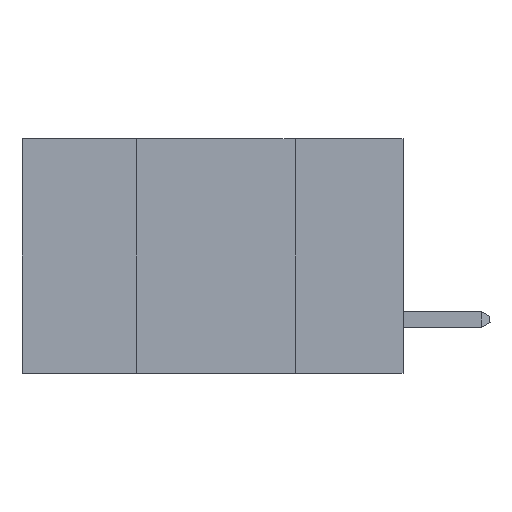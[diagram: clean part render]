
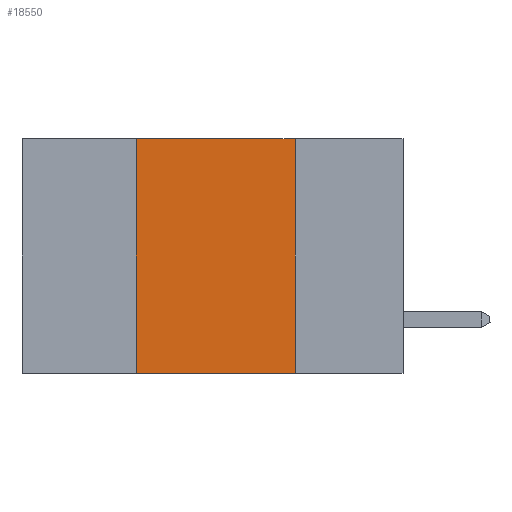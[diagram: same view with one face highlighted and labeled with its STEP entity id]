
A CAD part, left-side view. The second image highlights one B-rep face of the part: STEP entity #18550.
In plain terms, the highlighted planar face has unit normal (-1, 0, 0).
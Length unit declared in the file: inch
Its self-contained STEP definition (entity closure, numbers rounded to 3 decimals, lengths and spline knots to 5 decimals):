
#1432 = CARTESIAN_POINT ( 'NONE',  ( 0., 0.42, -0.37 ) ) ;
#1629 = LINE ( 'NONE', #10689, #16198 ) ;
#2350 = VECTOR ( 'NONE', #7795, 39.37008 ) ;
#4616 = FACE_OUTER_BOUND ( 'NONE', #24418, .T. ) ;
#4777 = DIRECTION ( 'NONE',  ( 0., -1., 0. ) ) ;
#5772 = CARTESIAN_POINT ( 'NONE',  ( 0., 0.17, 0. ) ) ;
#6080 = CARTESIAN_POINT ( 'NONE',  ( 0., 0.42, 0. ) ) ;
#7795 = DIRECTION ( 'NONE',  ( 0., 0., -1. ) ) ;
#7841 = VERTEX_POINT ( 'NONE', #17746 ) ;
#8073 = ORIENTED_EDGE ( 'NONE', *, *, #16523, .F. ) ;
#8170 = DIRECTION ( 'NONE',  ( 0., -1., 0. ) ) ;
#8856 = VERTEX_POINT ( 'NONE', #9450 ) ;
#9450 = CARTESIAN_POINT ( 'NONE',  ( 0., 0.17, 0. ) ) ;
#9518 = VECTOR ( 'NONE', #8170, 39.37008 ) ;
#10583 = DIRECTION ( 'NONE',  ( 0., 0., 1. ) ) ;
#10689 = CARTESIAN_POINT ( 'NONE',  ( 0., 0.6, -0.37 ) ) ;
#11296 = PLANE ( 'NONE',  #26279 ) ;
#13311 = DIRECTION ( 'NONE',  ( 1., 0., 0. ) ) ;
#13578 = DIRECTION ( 'NONE',  ( 0., 0., -1. ) ) ;
#14227 = CARTESIAN_POINT ( 'NONE',  ( 0., 0.6, 0. ) ) ;
#14898 = CARTESIAN_POINT ( 'NONE',  ( 0., 0.42, 0. ) ) ;
#16198 = VECTOR ( 'NONE', #4777, 39.37008 ) ;
#16250 = LINE ( 'NONE', #5772, #2350 ) ;
#16523 = EDGE_CURVE ( 'NONE', #19482, #25799, #20253, .T. ) ;
#17116 = EDGE_CURVE ( 'NONE', #8856, #7841, #16250, .T. ) ;
#17746 = CARTESIAN_POINT ( 'NONE',  ( 0., 0.17, -0.37 ) ) ;
#17961 = EDGE_CURVE ( 'NONE', #19482, #7841, #1629, .T. ) ;
#18550 = ADVANCED_FACE ( 'NONE', ( #4616 ), #11296, .F. ) ;
#19358 = ORIENTED_EDGE ( 'NONE', *, *, #17961, .T. ) ;
#19482 = VERTEX_POINT ( 'NONE', #1432 ) ;
#19576 = VECTOR ( 'NONE', #10583, 39.37008 ) ;
#20253 = LINE ( 'NONE', #14898, #19576 ) ;
#21857 = CARTESIAN_POINT ( 'NONE',  ( 0., 0.6, 0. ) ) ;
#24341 = EDGE_CURVE ( 'NONE', #25799, #8856, #27379, .T. ) ;
#24418 = EDGE_LOOP ( 'NONE', ( #24678, #25295, #8073, #19358 ) ) ;
#24678 = ORIENTED_EDGE ( 'NONE', *, *, #17116, .F. ) ;
#25295 = ORIENTED_EDGE ( 'NONE', *, *, #24341, .F. ) ;
#25799 = VERTEX_POINT ( 'NONE', #6080 ) ;
#26279 = AXIS2_PLACEMENT_3D ( 'NONE', #21857, #13311, #13578 ) ;
#27379 = LINE ( 'NONE', #14227, #9518 ) ;
